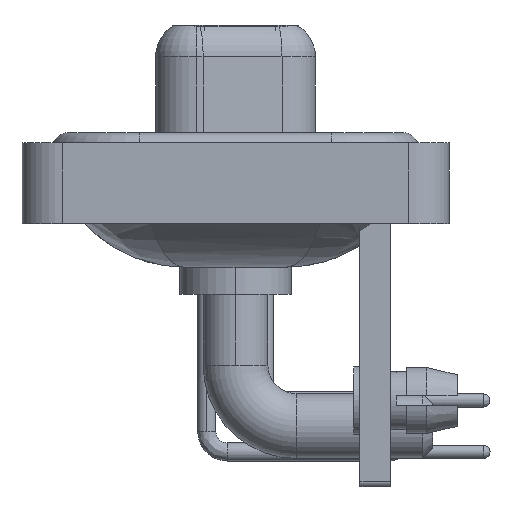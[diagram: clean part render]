
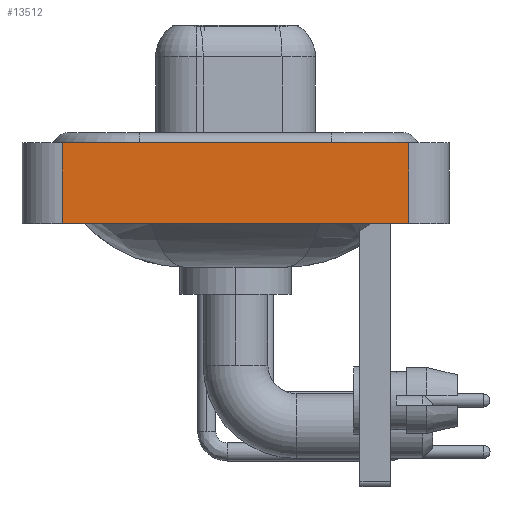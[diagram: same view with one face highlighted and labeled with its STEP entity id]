
A CAD part, left-side view. The second image highlights one B-rep face of the part: STEP entity #13512.
In plain terms, the highlighted planar face has unit normal (-1, 0, 0).
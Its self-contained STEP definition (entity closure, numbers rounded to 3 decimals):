
#707 = ORIENTED_EDGE ( 'NONE', *, *, #20198, .T. ) ;
#889 = ORIENTED_EDGE ( 'NONE', *, *, #18045, .F. ) ;
#980 = CARTESIAN_POINT ( 'NONE',  ( -7.35, -8.55, -3.6 ) ) ;
#2656 = DIRECTION ( 'NONE',  ( -1., 0., 0. ) ) ;
#3227 = CARTESIAN_POINT ( 'NONE',  ( -7.35, -8.55, 0.4 ) ) ;
#4194 = LINE ( 'NONE', #11974, #12638 ) ;
#4576 = DIRECTION ( 'NONE',  ( 0., 0., 1. ) ) ;
#6591 = LINE ( 'NONE', #20387, #21238 ) ;
#6701 = LINE ( 'NONE', #12435, #13208 ) ;
#6854 = VERTEX_POINT ( 'NONE', #23944 ) ;
#7129 = CARTESIAN_POINT ( 'NONE',  ( -7.35, -8.55, -3.6 ) ) ;
#7526 = VERTEX_POINT ( 'NONE', #3227 ) ;
#7992 = ORIENTED_EDGE ( 'NONE', *, *, #18560, .T. ) ;
#8195 = AXIS2_PLACEMENT_3D ( 'NONE', #980, #2656, #4576 ) ;
#9274 = CARTESIAN_POINT ( 'NONE',  ( -7.35, 8.55, -3.6 ) ) ;
#10292 = FACE_OUTER_BOUND ( 'NONE', #22975, .T. ) ;
#11974 = CARTESIAN_POINT ( 'NONE',  ( -7.35, -8.55, -3.6 ) ) ;
#12435 = CARTESIAN_POINT ( 'NONE',  ( -7.35, 8.55, -3.6 ) ) ;
#12638 = VECTOR ( 'NONE', #19791, 1000. ) ;
#12928 = CARTESIAN_POINT ( 'NONE',  ( -7.35, -8.55, -3.6 ) ) ;
#13208 = VECTOR ( 'NONE', #20129, 1000. ) ;
#13512 = ADVANCED_FACE ( 'NONE', ( #10292 ), #24235, .T. ) ;
#13906 = VERTEX_POINT ( 'NONE', #7129 ) ;
#13968 = VECTOR ( 'NONE', #17289, 1000. ) ;
#14873 = ORIENTED_EDGE ( 'NONE', *, *, #22210, .F. ) ;
#17289 = DIRECTION ( 'NONE',  ( 0., 0., 1. ) ) ;
#17732 = VERTEX_POINT ( 'NONE', #9274 ) ;
#18045 = EDGE_CURVE ( 'NONE', #6854, #7526, #6591, .T. ) ;
#18560 = EDGE_CURVE ( 'NONE', #13906, #7526, #19089, .T. ) ;
#18860 = DIRECTION ( 'NONE',  ( 0., -1., 0. ) ) ;
#19089 = LINE ( 'NONE', #12928, #13968 ) ;
#19791 = DIRECTION ( 'NONE',  ( 0., -1., 0. ) ) ;
#20129 = DIRECTION ( 'NONE',  ( 0., 0., 1. ) ) ;
#20198 = EDGE_CURVE ( 'NONE', #17732, #13906, #4194, .T. ) ;
#20387 = CARTESIAN_POINT ( 'NONE',  ( -7.35, -8.55, 0.4 ) ) ;
#21238 = VECTOR ( 'NONE', #18860, 1000. ) ;
#22210 = EDGE_CURVE ( 'NONE', #17732, #6854, #6701, .T. ) ;
#22975 = EDGE_LOOP ( 'NONE', ( #7992, #889, #14873, #707 ) ) ;
#23944 = CARTESIAN_POINT ( 'NONE',  ( -7.35, 8.55, 0.4 ) ) ;
#24235 = PLANE ( 'NONE',  #8195 ) ;
